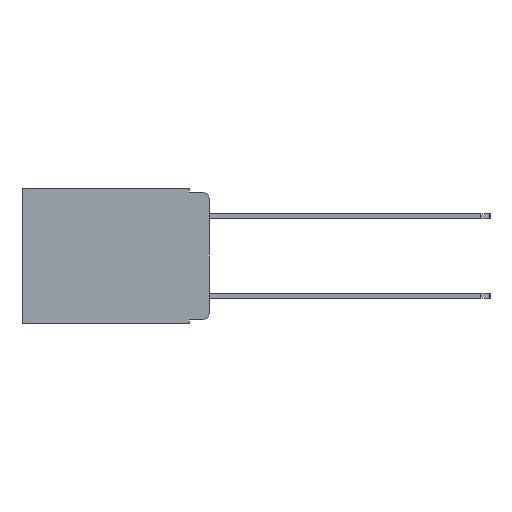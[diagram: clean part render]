
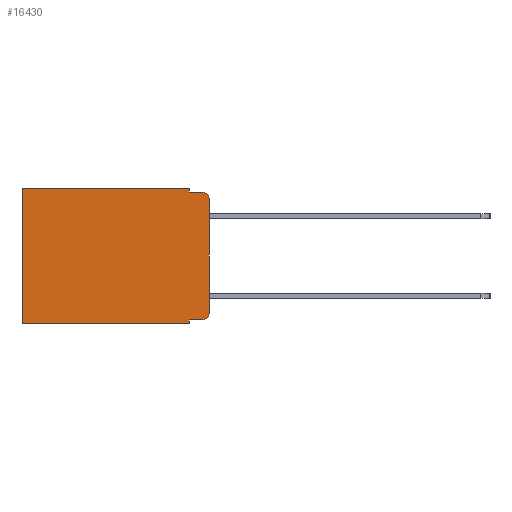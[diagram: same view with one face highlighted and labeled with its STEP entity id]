
A CAD part, left-side view. The second image highlights one B-rep face of the part: STEP entity #16430.
In plain terms, the highlighted planar face has unit normal (-1, 0, 0).
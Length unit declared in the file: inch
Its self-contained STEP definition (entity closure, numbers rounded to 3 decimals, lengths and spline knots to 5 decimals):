
#119 = ORIENTED_EDGE ( 'NONE', *, *, #3152, .T. ) ;
#149 = AXIS2_PLACEMENT_3D ( 'NONE', #1024, #10456, #2435 ) ;
#237 = DIRECTION ( 'NONE',  ( 0., 0., -1. ) ) ;
#331 = DIRECTION ( 'NONE',  ( 0., 0., -1. ) ) ;
#632 = VERTEX_POINT ( 'NONE', #11732 ) ;
#851 = EDGE_CURVE ( 'NONE', #11169, #7873, #4364, .T. ) ;
#1024 = CARTESIAN_POINT ( 'NONE',  ( 0.298, 0.02, -0.03 ) ) ;
#1089 = VECTOR ( 'NONE', #11034, 39.37008 ) ;
#1151 = CARTESIAN_POINT ( 'NONE',  ( 0.298, 0., -0.343 ) ) ;
#2363 = EDGE_CURVE ( 'NONE', #11169, #6137, #8314, .T. ) ;
#2435 = DIRECTION ( 'NONE',  ( 0., 0., -1. ) ) ;
#2698 = CARTESIAN_POINT ( 'NONE',  ( 0.298, 0.051, -0.333 ) ) ;
#2731 = ORIENTED_EDGE ( 'NONE', *, *, #15297, .F. ) ;
#2924 = DIRECTION ( 'NONE',  ( -1., 0., 0. ) ) ;
#2999 = VERTEX_POINT ( 'NONE', #16250 ) ;
#3152 = EDGE_CURVE ( 'NONE', #9771, #2999, #15817, .T. ) ;
#4130 = LINE ( 'NONE', #16478, #14385 ) ;
#4198 = ORIENTED_EDGE ( 'NONE', *, *, #5556, .T. ) ;
#4362 = VECTOR ( 'NONE', #17441, 39.37008 ) ;
#4364 = LINE ( 'NONE', #2698, #14218 ) ;
#4457 = EDGE_LOOP ( 'NONE', ( #5654, #14259, #5443, #2731, #119, #4198, #11529, #9224, #5081, #8486 ) ) ;
#4467 = DIRECTION ( 'NONE',  ( 0., -1., 0. ) ) ;
#4993 = CARTESIAN_POINT ( 'NONE',  ( 0.298, 0.473, 0. ) ) ;
#5081 = ORIENTED_EDGE ( 'NONE', *, *, #851, .T. ) ;
#5443 = ORIENTED_EDGE ( 'NONE', *, *, #10859, .F. ) ;
#5556 = EDGE_CURVE ( 'NONE', #2999, #10524, #5883, .T. ) ;
#5635 = CARTESIAN_POINT ( 'NONE',  ( 0.298, 0., 0. ) ) ;
#5654 = ORIENTED_EDGE ( 'NONE', *, *, #7256, .F. ) ;
#5883 = LINE ( 'NONE', #4993, #16601 ) ;
#6137 = VERTEX_POINT ( 'NONE', #7614 ) ;
#6506 = VERTEX_POINT ( 'NONE', #6512 ) ;
#6512 = CARTESIAN_POINT ( 'NONE',  ( 0.298, 0.02, -0.01 ) ) ;
#6889 = CIRCLE ( 'NONE', #10080, 0.02 ) ;
#7256 = EDGE_CURVE ( 'NONE', #14933, #632, #13800, .T. ) ;
#7269 = VECTOR ( 'NONE', #4467, 39.37008 ) ;
#7614 = CARTESIAN_POINT ( 'NONE',  ( 0.298, 0.051, -0.343 ) ) ;
#7873 = VERTEX_POINT ( 'NONE', #9368 ) ;
#8114 = CARTESIAN_POINT ( 'NONE',  ( 0.298, 0., 0. ) ) ;
#8314 = LINE ( 'NONE', #16531, #1089 ) ;
#8365 = DIRECTION ( 'NONE',  ( 1., 0., 0. ) ) ;
#8486 = ORIENTED_EDGE ( 'NONE', *, *, #9469, .T. ) ;
#8522 = FACE_OUTER_BOUND ( 'NONE', #4457, .T. ) ;
#8691 = VECTOR ( 'NONE', #16892, 39.37008 ) ;
#9224 = ORIENTED_EDGE ( 'NONE', *, *, #2363, .F. ) ;
#9368 = CARTESIAN_POINT ( 'NONE',  ( 0.298, 0.02, -0.333 ) ) ;
#9469 = EDGE_CURVE ( 'NONE', #7873, #632, #6889, .T. ) ;
#9542 = LINE ( 'NONE', #1151, #16680 ) ;
#9771 = VERTEX_POINT ( 'NONE', #15627 ) ;
#10080 = AXIS2_PLACEMENT_3D ( 'NONE', #10959, #2924, #12312 ) ;
#10441 = VERTEX_POINT ( 'NONE', #17041 ) ;
#10456 = DIRECTION ( 'NONE',  ( -1., 0., 0. ) ) ;
#10524 = VERTEX_POINT ( 'NONE', #17155 ) ;
#10859 = EDGE_CURVE ( 'NONE', #10441, #6506, #13993, .T. ) ;
#10959 = CARTESIAN_POINT ( 'NONE',  ( 0.298, 0.02, -0.313 ) ) ;
#11034 = DIRECTION ( 'NONE',  ( 0., 0., -1. ) ) ;
#11152 = CARTESIAN_POINT ( 'NONE',  ( 0.298, 0.051, -0.01 ) ) ;
#11169 = VERTEX_POINT ( 'NONE', #15642 ) ;
#11529 = ORIENTED_EDGE ( 'NONE', *, *, #12209, .F. ) ;
#11709 = EDGE_CURVE ( 'NONE', #14933, #6506, #14375, .T. ) ;
#11732 = CARTESIAN_POINT ( 'NONE',  ( 0.298, 0., -0.313 ) ) ;
#11964 = DIRECTION ( 'NONE',  ( 0., 1., 0. ) ) ;
#12209 = EDGE_CURVE ( 'NONE', #6137, #10524, #9542, .T. ) ;
#12312 = DIRECTION ( 'NONE',  ( 0., 0., -1. ) ) ;
#12522 = CARTESIAN_POINT ( 'NONE',  ( 0.298, 0., -0.03 ) ) ;
#13800 = LINE ( 'NONE', #8114, #4362 ) ;
#13993 = LINE ( 'NONE', #11152, #7269 ) ;
#14218 = VECTOR ( 'NONE', #17048, 39.37008 ) ;
#14259 = ORIENTED_EDGE ( 'NONE', *, *, #11709, .T. ) ;
#14375 = CIRCLE ( 'NONE', #149, 0.02 ) ;
#14382 = DIRECTION ( 'NONE',  ( 0., 0., -1. ) ) ;
#14385 = VECTOR ( 'NONE', #331, 39.37008 ) ;
#14933 = VERTEX_POINT ( 'NONE', #12522 ) ;
#15297 = EDGE_CURVE ( 'NONE', #9771, #10441, #4130, .T. ) ;
#15627 = CARTESIAN_POINT ( 'NONE',  ( 0.298, 0.051, 0. ) ) ;
#15642 = CARTESIAN_POINT ( 'NONE',  ( 0.298, 0.051, -0.333 ) ) ;
#15817 = LINE ( 'NONE', #16954, #8691 ) ;
#16250 = CARTESIAN_POINT ( 'NONE',  ( 0.298, 0.473, 0. ) ) ;
#16380 = PLANE ( 'NONE',  #16986 ) ;
#16430 = ADVANCED_FACE ( 'NONE', ( #8522 ), #16380, .F. ) ;
#16478 = CARTESIAN_POINT ( 'NONE',  ( 0.298, 0.051, 0. ) ) ;
#16531 = CARTESIAN_POINT ( 'NONE',  ( 0.298, 0.051, 0. ) ) ;
#16601 = VECTOR ( 'NONE', #14382, 39.37008 ) ;
#16680 = VECTOR ( 'NONE', #11964, 39.37008 ) ;
#16892 = DIRECTION ( 'NONE',  ( 0., 1., 0. ) ) ;
#16954 = CARTESIAN_POINT ( 'NONE',  ( 0.298, 0., 0. ) ) ;
#16986 = AXIS2_PLACEMENT_3D ( 'NONE', #5635, #8365, #237 ) ;
#17041 = CARTESIAN_POINT ( 'NONE',  ( 0.298, 0.051, -0.01 ) ) ;
#17048 = DIRECTION ( 'NONE',  ( 0., -1., 0. ) ) ;
#17155 = CARTESIAN_POINT ( 'NONE',  ( 0.298, 0.473, -0.343 ) ) ;
#17441 = DIRECTION ( 'NONE',  ( 0., 0., -1. ) ) ;
